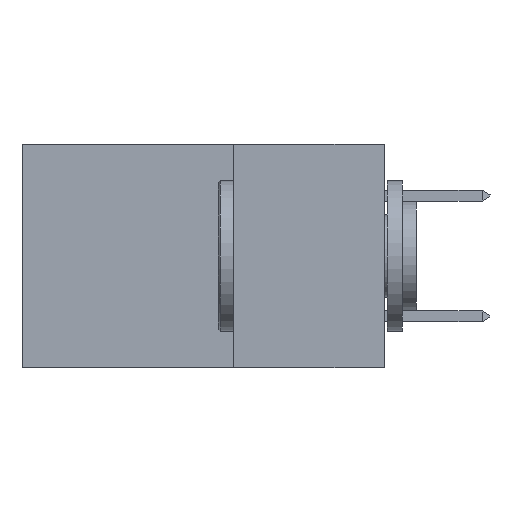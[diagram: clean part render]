
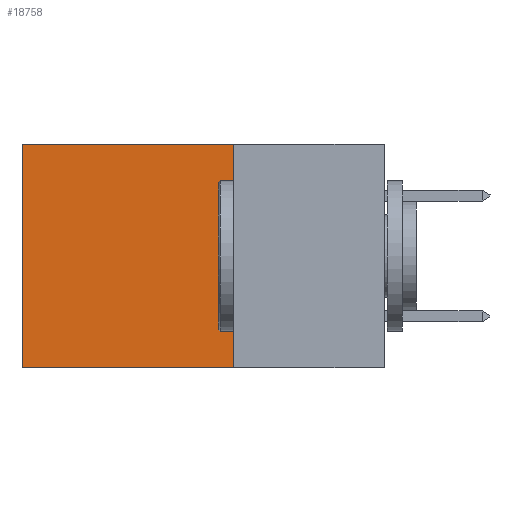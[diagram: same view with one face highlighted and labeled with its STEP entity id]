
A CAD part, left-side view. The second image highlights one B-rep face of the part: STEP entity #18758.
In plain terms, the highlighted planar face has unit normal (-1, 0, 0).
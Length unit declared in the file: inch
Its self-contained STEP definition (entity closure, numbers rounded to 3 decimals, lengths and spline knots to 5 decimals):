
#1254 = FACE_OUTER_BOUND ( 'NONE', #40094, .T. ) ;
#2094 = VERTEX_POINT ( 'NONE', #41227 ) ;
#2472 = LINE ( 'NONE', #4977, #9116 ) ;
#2507 = LINE ( 'NONE', #28184, #33084 ) ;
#2582 = DIRECTION ( 'NONE',  ( 0., 0., -1. ) ) ;
#4977 = CARTESIAN_POINT ( 'NONE',  ( 0.2875, 0.6, 0. ) ) ;
#5098 = ORIENTED_EDGE ( 'NONE', *, *, #5616, .T. ) ;
#5616 = EDGE_CURVE ( 'NONE', #41329, #20562, #25322, .T. ) ;
#5881 = CARTESIAN_POINT ( 'NONE',  ( 0.2875, 0.25, 0. ) ) ;
#8564 = DIRECTION ( 'NONE',  ( 0., 0., -1. ) ) ;
#9116 = VECTOR ( 'NONE', #8564, 39.37008 ) ;
#9294 = PLANE ( 'NONE',  #24602 ) ;
#9573 = EDGE_CURVE ( 'NONE', #39838, #2094, #2507, .T. ) ;
#13323 = CARTESIAN_POINT ( 'NONE',  ( 0.2875, 0.25, -0.37 ) ) ;
#16007 = CARTESIAN_POINT ( 'NONE',  ( 0.2875, 0.25, 0. ) ) ;
#18758 = ADVANCED_FACE ( 'NONE', ( #1254 ), #9294, .F. ) ;
#20562 = VERTEX_POINT ( 'NONE', #37577 ) ;
#23178 = EDGE_CURVE ( 'NONE', #20562, #2094, #2472, .T. ) ;
#23523 = DIRECTION ( 'NONE',  ( 0., 0., -1. ) ) ;
#24574 = CARTESIAN_POINT ( 'NONE',  ( 0.2875, 0.25, 0. ) ) ;
#24602 = AXIS2_PLACEMENT_3D ( 'NONE', #35090, #35375, #2582 ) ;
#25322 = LINE ( 'NONE', #5881, #27845 ) ;
#27845 = VECTOR ( 'NONE', #28703, 39.37008 ) ;
#28184 = CARTESIAN_POINT ( 'NONE',  ( 0.2875, 0.25, -0.37 ) ) ;
#28472 = ORIENTED_EDGE ( 'NONE', *, *, #23178, .T. ) ;
#28703 = DIRECTION ( 'NONE',  ( 0., 1., 0. ) ) ;
#31793 = VECTOR ( 'NONE', #23523, 39.37008 ) ;
#33084 = VECTOR ( 'NONE', #40790, 39.37008 ) ;
#35090 = CARTESIAN_POINT ( 'NONE',  ( 0.2875, 0.25, 0. ) ) ;
#35375 = DIRECTION ( 'NONE',  ( 1., 0., 0. ) ) ;
#37374 = ORIENTED_EDGE ( 'NONE', *, *, #9573, .F. ) ;
#37577 = CARTESIAN_POINT ( 'NONE',  ( 0.2875, 0.6, 0. ) ) ;
#39838 = VERTEX_POINT ( 'NONE', #13323 ) ;
#40094 = EDGE_LOOP ( 'NONE', ( #28472, #37374, #40115, #5098 ) ) ;
#40115 = ORIENTED_EDGE ( 'NONE', *, *, #40554, .F. ) ;
#40380 = LINE ( 'NONE', #16007, #31793 ) ;
#40554 = EDGE_CURVE ( 'NONE', #41329, #39838, #40380, .T. ) ;
#40790 = DIRECTION ( 'NONE',  ( 0., 1., 0. ) ) ;
#41227 = CARTESIAN_POINT ( 'NONE',  ( 0.2875, 0.6, -0.37 ) ) ;
#41329 = VERTEX_POINT ( 'NONE', #24574 ) ;
